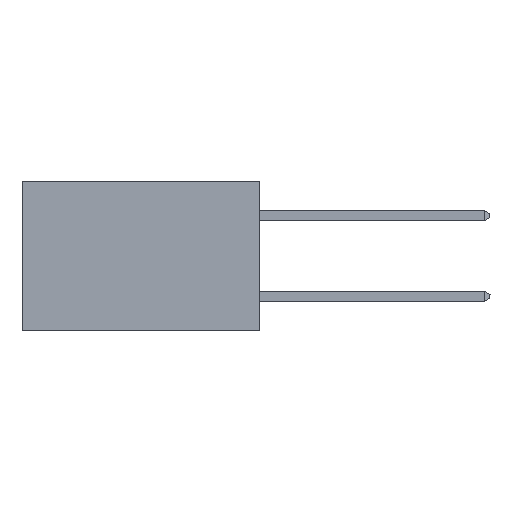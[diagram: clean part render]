
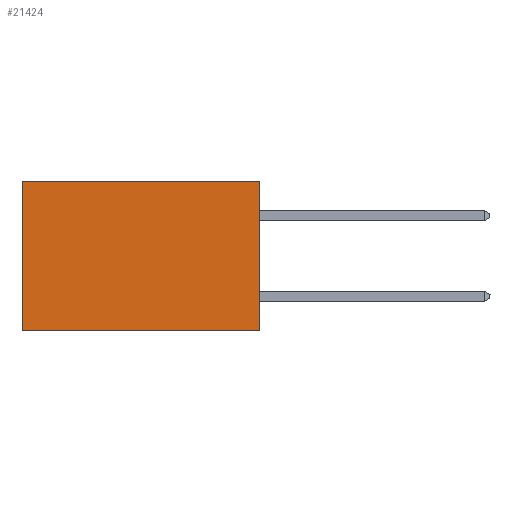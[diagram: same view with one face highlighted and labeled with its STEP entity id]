
A CAD part, left-side view. The second image highlights one B-rep face of the part: STEP entity #21424.
In plain terms, the highlighted planar face has unit normal (-1, 0, 0).
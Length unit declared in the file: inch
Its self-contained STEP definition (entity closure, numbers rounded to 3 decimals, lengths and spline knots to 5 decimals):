
#166 = LINE ( 'NONE', #16980, #11600 ) ;
#215 = VECTOR ( 'NONE', #2968, 39.37008 ) ;
#929 = VECTOR ( 'NONE', #8561, 39.37008 ) ;
#2742 = VERTEX_POINT ( 'NONE', #21514 ) ;
#2968 = DIRECTION ( 'NONE',  ( 0., 0., -1. ) ) ;
#3392 = AXIS2_PLACEMENT_3D ( 'NONE', #8722, #11014, #26704 ) ;
#5571 = LINE ( 'NONE', #13463, #28752 ) ;
#5621 = CARTESIAN_POINT ( 'NONE',  ( 0.277, 0., 0. ) ) ;
#6436 = EDGE_CURVE ( 'NONE', #16140, #20421, #16911, .T. ) ;
#7309 = ORIENTED_EDGE ( 'NONE', *, *, #20857, .F. ) ;
#7323 = EDGE_CURVE ( 'NONE', #16140, #28542, #166, .T. ) ;
#8561 = DIRECTION ( 'NONE',  ( 0., 0., -1. ) ) ;
#8722 = CARTESIAN_POINT ( 'NONE',  ( 0.277, 0., -0.37 ) ) ;
#9458 = ORIENTED_EDGE ( 'NONE', *, *, #6436, .F. ) ;
#11014 = DIRECTION ( 'NONE',  ( 1., 0., 0. ) ) ;
#11241 = EDGE_LOOP ( 'NONE', ( #16896, #7309, #9458, #18957 ) ) ;
#11600 = VECTOR ( 'NONE', #19241, 39.37008 ) ;
#12812 = CARTESIAN_POINT ( 'NONE',  ( 0.277, 0.59, 0. ) ) ;
#13463 = CARTESIAN_POINT ( 'NONE',  ( 0.277, 0., -0.37 ) ) ;
#16140 = VERTEX_POINT ( 'NONE', #5621 ) ;
#16896 = ORIENTED_EDGE ( 'NONE', *, *, #27165, .T. ) ;
#16911 = LINE ( 'NONE', #25486, #215 ) ;
#16980 = CARTESIAN_POINT ( 'NONE',  ( 0.277, 0., 0. ) ) ;
#17376 = DIRECTION ( 'NONE',  ( 0., 1., 0. ) ) ;
#18957 = ORIENTED_EDGE ( 'NONE', *, *, #7323, .T. ) ;
#19241 = DIRECTION ( 'NONE',  ( 0., 1., 0. ) ) ;
#20421 = VERTEX_POINT ( 'NONE', #23128 ) ;
#20857 = EDGE_CURVE ( 'NONE', #20421, #2742, #5571, .T. ) ;
#21424 = ADVANCED_FACE ( 'NONE', ( #26645 ), #22211, .F. ) ;
#21514 = CARTESIAN_POINT ( 'NONE',  ( 0.277, 0.59, -0.37 ) ) ;
#22211 = PLANE ( 'NONE',  #3392 ) ;
#23128 = CARTESIAN_POINT ( 'NONE',  ( 0.277, 0., -0.37 ) ) ;
#24395 = CARTESIAN_POINT ( 'NONE',  ( 0.277, 0.59, -0.37 ) ) ;
#25008 = LINE ( 'NONE', #24395, #929 ) ;
#25486 = CARTESIAN_POINT ( 'NONE',  ( 0.277, 0., -0.37 ) ) ;
#26645 = FACE_OUTER_BOUND ( 'NONE', #11241, .T. ) ;
#26704 = DIRECTION ( 'NONE',  ( 0., 0., -1. ) ) ;
#27165 = EDGE_CURVE ( 'NONE', #28542, #2742, #25008, .T. ) ;
#28542 = VERTEX_POINT ( 'NONE', #12812 ) ;
#28752 = VECTOR ( 'NONE', #17376, 39.37008 ) ;
